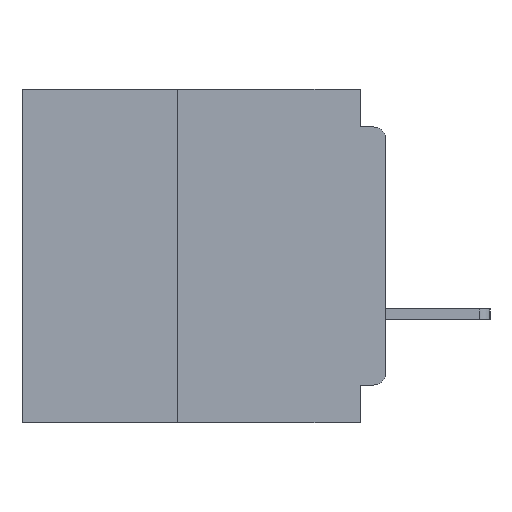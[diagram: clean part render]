
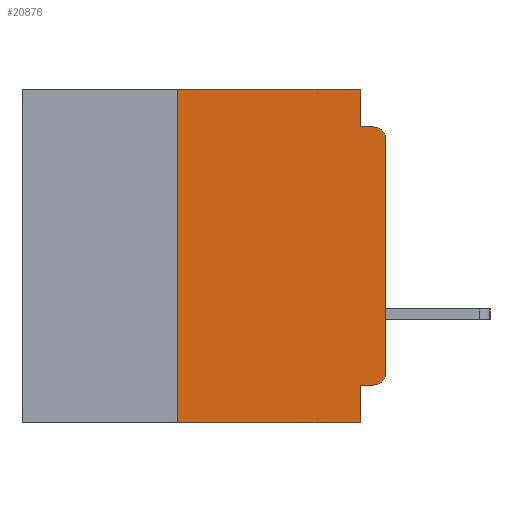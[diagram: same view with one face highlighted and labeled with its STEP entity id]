
A CAD part, left-side view. The second image highlights one B-rep face of the part: STEP entity #20876.
In plain terms, the highlighted planar face has unit normal (-1, 0, 0).
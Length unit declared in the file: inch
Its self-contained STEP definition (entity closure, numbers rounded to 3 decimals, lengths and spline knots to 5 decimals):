
#62 = AXIS2_PLACEMENT_3D ( 'NONE', #12834, #39490, #16735 ) ;
#1098 = CARTESIAN_POINT ( 'NONE',  ( 0., 0.437, -0.4 ) ) ;
#1467 = DIRECTION ( 'NONE',  ( 0., -1., 0. ) ) ;
#2306 = CARTESIAN_POINT ( 'NONE',  ( 0., 0.031, -0.355 ) ) ;
#2580 = VERTEX_POINT ( 'NONE', #3366 ) ;
#2969 = EDGE_CURVE ( 'NONE', #5013, #5351, #21031, .T. ) ;
#3366 = CARTESIAN_POINT ( 'NONE',  ( 0., 0., -0.06 ) ) ;
#3965 = CARTESIAN_POINT ( 'NONE',  ( 0., 0.015, -0.355 ) ) ;
#4301 = CIRCLE ( 'NONE', #62, 0.015 ) ;
#4448 = VECTOR ( 'NONE', #16582, 39.37008 ) ;
#4999 = ORIENTED_EDGE ( 'NONE', *, *, #35223, .F. ) ;
#5013 = VERTEX_POINT ( 'NONE', #22106 ) ;
#5351 = VERTEX_POINT ( 'NONE', #42851 ) ;
#5537 = CARTESIAN_POINT ( 'NONE',  ( 0., 0.015, -0.34 ) ) ;
#5963 = PLANE ( 'NONE',  #31015 ) ;
#9417 = EDGE_CURVE ( 'NONE', #17549, #25013, #45284, .T. ) ;
#9470 = DIRECTION ( 'NONE',  ( 0., 0., -1. ) ) ;
#10037 = CARTESIAN_POINT ( 'NONE',  ( 0., 0.25, -0.4 ) ) ;
#10171 = VERTEX_POINT ( 'NONE', #36515 ) ;
#10806 = VECTOR ( 'NONE', #18055, 39.37008 ) ;
#11739 = AXIS2_PLACEMENT_3D ( 'NONE', #5537, #32312, #9470 ) ;
#11785 = ORIENTED_EDGE ( 'NONE', *, *, #9417, .F. ) ;
#12076 = DIRECTION ( 'NONE',  ( 0., 0., -1. ) ) ;
#12147 = CARTESIAN_POINT ( 'NONE',  ( 0., 0., -0.34 ) ) ;
#12194 = EDGE_CURVE ( 'NONE', #42084, #2580, #36679, .T. ) ;
#12681 = CARTESIAN_POINT ( 'NONE',  ( 0., 0., -0.355 ) ) ;
#12834 = CARTESIAN_POINT ( 'NONE',  ( 0., 0.015, -0.06 ) ) ;
#12977 = ORIENTED_EDGE ( 'NONE', *, *, #39449, .T. ) ;
#13772 = DIRECTION ( 'NONE',  ( 0., 0., -1. ) ) ;
#16300 = EDGE_CURVE ( 'NONE', #10171, #5013, #47652, .T. ) ;
#16582 = DIRECTION ( 'NONE',  ( 0., 1., 0. ) ) ;
#16735 = DIRECTION ( 'NONE',  ( 0., 0., -1. ) ) ;
#17549 = VERTEX_POINT ( 'NONE', #2306 ) ;
#18055 = DIRECTION ( 'NONE',  ( 0., -1., 0. ) ) ;
#19068 = LINE ( 'NONE', #1098, #28008 ) ;
#19668 = CARTESIAN_POINT ( 'NONE',  ( 0., 0.031, -0.4 ) ) ;
#19894 = VERTEX_POINT ( 'NONE', #35788 ) ;
#20530 = EDGE_LOOP ( 'NONE', ( #39467, #36910, #45026, #34175, #4999, #46292, #36439, #11785, #25003, #12977 ) ) ;
#20585 = CARTESIAN_POINT ( 'NONE',  ( 0., 0.25, 0. ) ) ;
#20876 = ADVANCED_FACE ( 'NONE', ( #41710 ), #5963, .F. ) ;
#21031 = LINE ( 'NONE', #33128, #10806 ) ;
#21683 = CARTESIAN_POINT ( 'NONE',  ( 0., 0.031, -0.4 ) ) ;
#22106 = CARTESIAN_POINT ( 'NONE',  ( 0., 0.031, -0.045 ) ) ;
#23203 = EDGE_CURVE ( 'NONE', #42664, #17549, #32596, .T. ) ;
#24180 = DIRECTION ( 'NONE',  ( 0., -1., 0. ) ) ;
#24967 = DIRECTION ( 'NONE',  ( 0., 0., 1. ) ) ;
#25003 = ORIENTED_EDGE ( 'NONE', *, *, #23203, .F. ) ;
#25013 = VERTEX_POINT ( 'NONE', #21683 ) ;
#28008 = VECTOR ( 'NONE', #24180, 39.37008 ) ;
#28941 = CARTESIAN_POINT ( 'NONE',  ( 0., 0.437, 0. ) ) ;
#30450 = EDGE_CURVE ( 'NONE', #2580, #5351, #4301, .T. ) ;
#31015 = AXIS2_PLACEMENT_3D ( 'NONE', #28941, #36563, #13772 ) ;
#32072 = DIRECTION ( 'NONE',  ( 0., 0., -1. ) ) ;
#32312 = DIRECTION ( 'NONE',  ( -1., 0., 0. ) ) ;
#32596 = LINE ( 'NONE', #12681, #4448 ) ;
#32781 = VECTOR ( 'NONE', #12076, 39.37008 ) ;
#32784 = EDGE_CURVE ( 'NONE', #19894, #33239, #44966, .T. ) ;
#33128 = CARTESIAN_POINT ( 'NONE',  ( 0., 0., -0.045 ) ) ;
#33239 = VERTEX_POINT ( 'NONE', #20585 ) ;
#34175 = ORIENTED_EDGE ( 'NONE', *, *, #16300, .F. ) ;
#34823 = VECTOR ( 'NONE', #36728, 39.37008 ) ;
#35223 = EDGE_CURVE ( 'NONE', #33239, #10171, #37656, .T. ) ;
#35788 = CARTESIAN_POINT ( 'NONE',  ( 0., 0.25, -0.4 ) ) ;
#36439 = ORIENTED_EDGE ( 'NONE', *, *, #46788, .T. ) ;
#36515 = CARTESIAN_POINT ( 'NONE',  ( 0., 0.031, 0. ) ) ;
#36563 = DIRECTION ( 'NONE',  ( 1., 0., 0. ) ) ;
#36679 = LINE ( 'NONE', #47706, #46784 ) ;
#36728 = DIRECTION ( 'NONE',  ( 0., 0., 1. ) ) ;
#36910 = ORIENTED_EDGE ( 'NONE', *, *, #30450, .T. ) ;
#37532 = VECTOR ( 'NONE', #32072, 39.37008 ) ;
#37656 = LINE ( 'NONE', #47288, #46582 ) ;
#39449 = EDGE_CURVE ( 'NONE', #42664, #42084, #44492, .T. ) ;
#39467 = ORIENTED_EDGE ( 'NONE', *, *, #12194, .T. ) ;
#39490 = DIRECTION ( 'NONE',  ( -1., 0., 0. ) ) ;
#39557 = CARTESIAN_POINT ( 'NONE',  ( 0., 0.031, 0. ) ) ;
#41710 = FACE_OUTER_BOUND ( 'NONE', #20530, .T. ) ;
#42084 = VERTEX_POINT ( 'NONE', #12147 ) ;
#42664 = VERTEX_POINT ( 'NONE', #3965 ) ;
#42851 = CARTESIAN_POINT ( 'NONE',  ( 0., 0.015, -0.045 ) ) ;
#44492 = CIRCLE ( 'NONE', #11739, 0.015 ) ;
#44966 = LINE ( 'NONE', #10037, #34823 ) ;
#45026 = ORIENTED_EDGE ( 'NONE', *, *, #2969, .F. ) ;
#45284 = LINE ( 'NONE', #19668, #32781 ) ;
#46292 = ORIENTED_EDGE ( 'NONE', *, *, #32784, .F. ) ;
#46582 = VECTOR ( 'NONE', #1467, 39.37008 ) ;
#46784 = VECTOR ( 'NONE', #24967, 39.37008 ) ;
#46788 = EDGE_CURVE ( 'NONE', #19894, #25013, #19068, .T. ) ;
#47288 = CARTESIAN_POINT ( 'NONE',  ( 0., 0.437, 0. ) ) ;
#47652 = LINE ( 'NONE', #39557, #37532 ) ;
#47706 = CARTESIAN_POINT ( 'NONE',  ( 0., 0., 0. ) ) ;
